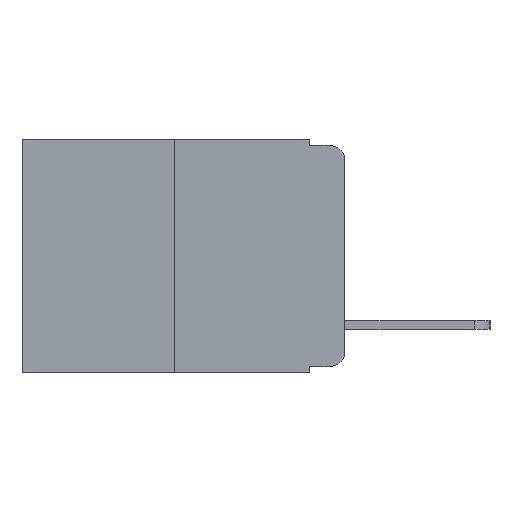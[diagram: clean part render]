
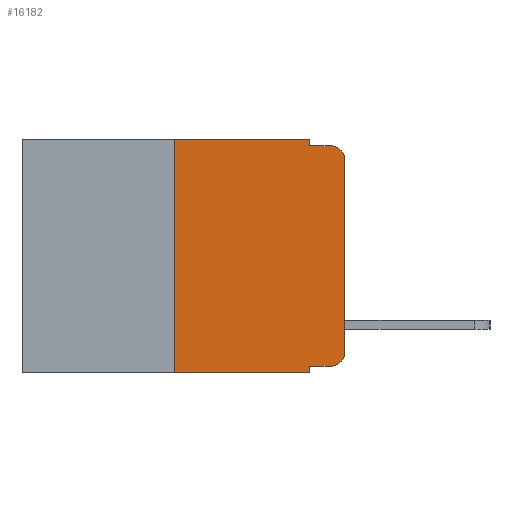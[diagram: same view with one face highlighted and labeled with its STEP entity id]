
A CAD part, left-side view. The second image highlights one B-rep face of the part: STEP entity #16182.
In plain terms, the highlighted planar face has unit normal (-1, 0, 0).
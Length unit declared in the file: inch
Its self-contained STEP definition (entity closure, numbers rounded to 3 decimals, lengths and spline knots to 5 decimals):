
#139 = CIRCLE ( 'NONE', #12214, 0.02 ) ;
#155 = LINE ( 'NONE', #3318, #13856 ) ;
#700 = VERTEX_POINT ( 'NONE', #7074 ) ;
#984 = VERTEX_POINT ( 'NONE', #13564 ) ;
#1095 = EDGE_CURVE ( 'NONE', #13029, #984, #13812, .T. ) ;
#1196 = CIRCLE ( 'NONE', #3152, 0.02 ) ;
#1438 = DIRECTION ( 'NONE',  ( 0., -1., 0. ) ) ;
#1466 = EDGE_CURVE ( 'NONE', #4967, #700, #8325, .T. ) ;
#1557 = VERTEX_POINT ( 'NONE', #4728 ) ;
#1640 = DIRECTION ( 'NONE',  ( 0., 0., -1. ) ) ;
#1643 = DIRECTION ( 'NONE',  ( -1., 0., 0. ) ) ;
#1668 = CARTESIAN_POINT ( 'NONE',  ( 0., 0.02, -0.313 ) ) ;
#2434 = VERTEX_POINT ( 'NONE', #12503 ) ;
#2597 = EDGE_CURVE ( 'NONE', #11667, #7537, #10380, .T. ) ;
#2809 = CARTESIAN_POINT ( 'NONE',  ( 0., 0.051, 0. ) ) ;
#3152 = AXIS2_PLACEMENT_3D ( 'NONE', #1668, #1643, #1640 ) ;
#3318 = CARTESIAN_POINT ( 'NONE',  ( 0., 0.051, -0.01 ) ) ;
#3745 = PLANE ( 'NONE',  #16328 ) ;
#4149 = VERTEX_POINT ( 'NONE', #16430 ) ;
#4266 = EDGE_CURVE ( 'NONE', #6985, #11667, #8786, .T. ) ;
#4525 = LINE ( 'NONE', #12921, #10680 ) ;
#4700 = LINE ( 'NONE', #10969, #7785 ) ;
#4728 = CARTESIAN_POINT ( 'NONE',  ( 0., 0.02, -0.01 ) ) ;
#4967 = VERTEX_POINT ( 'NONE', #5245 ) ;
#5245 = CARTESIAN_POINT ( 'NONE',  ( 0., 0.051, -0.333 ) ) ;
#5348 = VECTOR ( 'NONE', #13400, 39.37008 ) ;
#6484 = FACE_OUTER_BOUND ( 'NONE', #15785, .T. ) ;
#6985 = VERTEX_POINT ( 'NONE', #14718 ) ;
#7074 = CARTESIAN_POINT ( 'NONE',  ( 0., 0.02, -0.333 ) ) ;
#7365 = CARTESIAN_POINT ( 'NONE',  ( 0., 0.051, 0. ) ) ;
#7526 = VECTOR ( 'NONE', #13874, 39.37008 ) ;
#7537 = VERTEX_POINT ( 'NONE', #13494 ) ;
#7641 = EDGE_CURVE ( 'NONE', #4967, #984, #4525, .T. ) ;
#7785 = VECTOR ( 'NONE', #10952, 39.37008 ) ;
#8325 = LINE ( 'NONE', #13615, #14176 ) ;
#8786 = LINE ( 'NONE', #14410, #11436 ) ;
#9102 = DIRECTION ( 'NONE',  ( 0., 0., -1. ) ) ;
#9115 = DIRECTION ( 'NONE',  ( -1., 0., 0. ) ) ;
#9130 = CARTESIAN_POINT ( 'NONE',  ( 0., 0.02, -0.03 ) ) ;
#9619 = EDGE_CURVE ( 'NONE', #4149, #2434, #14918, .T. ) ;
#10003 = EDGE_CURVE ( 'NONE', #13029, #6985, #4700, .T. ) ;
#10312 = EDGE_CURVE ( 'NONE', #2434, #1557, #139, .T. ) ;
#10380 = LINE ( 'NONE', #7365, #13562 ) ;
#10680 = VECTOR ( 'NONE', #12020, 39.37008 ) ;
#10952 = DIRECTION ( 'NONE',  ( 0., 0., 1. ) ) ;
#10969 = CARTESIAN_POINT ( 'NONE',  ( 0., 0.25, 0. ) ) ;
#11068 = CARTESIAN_POINT ( 'NONE',  ( 0., 0.473, -0.343 ) ) ;
#11436 = VECTOR ( 'NONE', #14506, 39.37008 ) ;
#11667 = VERTEX_POINT ( 'NONE', #2809 ) ;
#11806 = EDGE_CURVE ( 'NONE', #700, #4149, #1196, .T. ) ;
#12020 = DIRECTION ( 'NONE',  ( 0., 0., -1. ) ) ;
#12214 = AXIS2_PLACEMENT_3D ( 'NONE', #9130, #9115, #9102 ) ;
#12503 = CARTESIAN_POINT ( 'NONE',  ( 0., 0., -0.03 ) ) ;
#12669 = EDGE_CURVE ( 'NONE', #7537, #1557, #155, .T. ) ;
#12710 = CARTESIAN_POINT ( 'NONE',  ( 0., 0.25, -0.343 ) ) ;
#12921 = CARTESIAN_POINT ( 'NONE',  ( 0., 0.051, 0. ) ) ;
#13029 = VERTEX_POINT ( 'NONE', #12710 ) ;
#13148 = DIRECTION ( 'NONE',  ( 1., 0., 0. ) ) ;
#13154 = CARTESIAN_POINT ( 'NONE',  ( 0., 0.473, 0. ) ) ;
#13400 = DIRECTION ( 'NONE',  ( 0., 0., 1. ) ) ;
#13494 = CARTESIAN_POINT ( 'NONE',  ( 0., 0.051, -0.01 ) ) ;
#13547 = CARTESIAN_POINT ( 'NONE',  ( 0., 0., 0. ) ) ;
#13562 = VECTOR ( 'NONE', #13998, 39.37008 ) ;
#13564 = CARTESIAN_POINT ( 'NONE',  ( 0., 0.051, -0.343 ) ) ;
#13615 = CARTESIAN_POINT ( 'NONE',  ( 0., 0.051, -0.333 ) ) ;
#13812 = LINE ( 'NONE', #11068, #7526 ) ;
#13856 = VECTOR ( 'NONE', #1438, 39.37008 ) ;
#13874 = DIRECTION ( 'NONE',  ( 0., -1., 0. ) ) ;
#13952 = ORIENTED_EDGE ( 'NONE', *, *, #9619, .T. ) ;
#13972 = ORIENTED_EDGE ( 'NONE', *, *, #10312, .T. ) ;
#13987 = ORIENTED_EDGE ( 'NONE', *, *, #12669, .F. ) ;
#13998 = DIRECTION ( 'NONE',  ( 0., 0., -1. ) ) ;
#14028 = ORIENTED_EDGE ( 'NONE', *, *, #2597, .F. ) ;
#14163 = ORIENTED_EDGE ( 'NONE', *, *, #4266, .F. ) ;
#14171 = ORIENTED_EDGE ( 'NONE', *, *, #10003, .F. ) ;
#14176 = VECTOR ( 'NONE', #14449, 39.37008 ) ;
#14326 = ORIENTED_EDGE ( 'NONE', *, *, #1095, .T. ) ;
#14410 = CARTESIAN_POINT ( 'NONE',  ( 0., 0.473, 0. ) ) ;
#14449 = DIRECTION ( 'NONE',  ( 0., -1., 0. ) ) ;
#14506 = DIRECTION ( 'NONE',  ( 0., -1., 0. ) ) ;
#14669 = ORIENTED_EDGE ( 'NONE', *, *, #7641, .F. ) ;
#14718 = CARTESIAN_POINT ( 'NONE',  ( 0., 0.25, 0. ) ) ;
#14918 = LINE ( 'NONE', #13547, #5348 ) ;
#15183 = ORIENTED_EDGE ( 'NONE', *, *, #1466, .T. ) ;
#15192 = ORIENTED_EDGE ( 'NONE', *, *, #11806, .T. ) ;
#15785 = EDGE_LOOP ( 'NONE', ( #13952, #13972, #13987, #14028, #14163, #14171, #14326, #14669, #15183, #15192 ) ) ;
#16182 = ADVANCED_FACE ( 'NONE', ( #6484 ), #3745, .F. ) ;
#16328 = AXIS2_PLACEMENT_3D ( 'NONE', #13154, #13148, #16518 ) ;
#16430 = CARTESIAN_POINT ( 'NONE',  ( 0., 0., -0.313 ) ) ;
#16518 = DIRECTION ( 'NONE',  ( 0., 0., -1. ) ) ;
